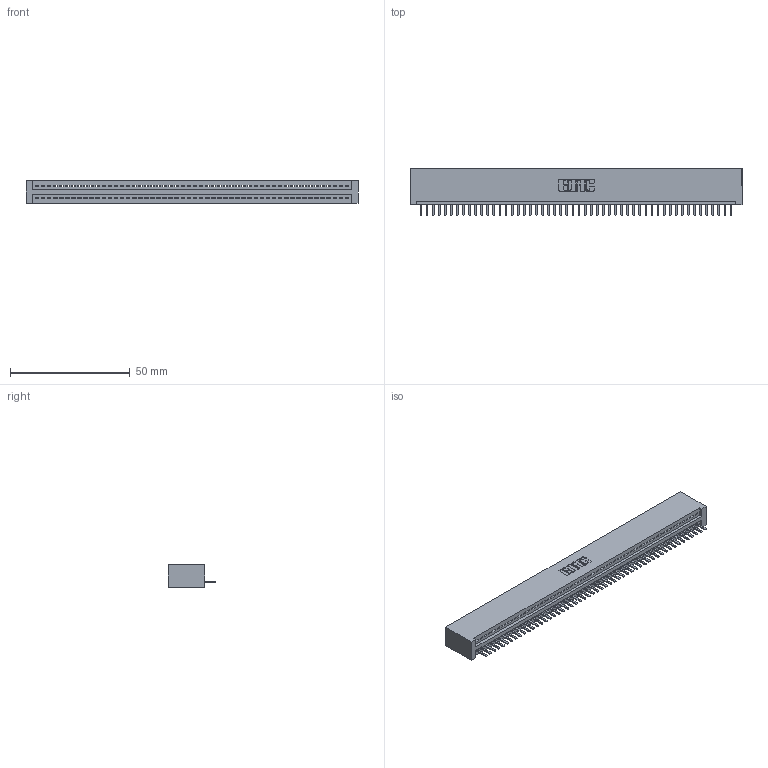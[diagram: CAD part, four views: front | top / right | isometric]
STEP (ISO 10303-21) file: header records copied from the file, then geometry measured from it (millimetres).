
FILE_DESCRIPTION (( 'STEP AP203' ), '1' );
FILE_NAME ('395-052-520-101.STEP', '2019-10-23T11:31:00', ( '' ), ( '' ), 'SwSTEP 2.0', 'SolidWorks 2016', '' );
FILE_SCHEMA (( 'CONFIG_CONTROL_DESIGN' ));
Length unit declared in the file: inch
Products named in the file (3): 345 Part_No Mounting Lugs; 395-052-520-101; 345-292-001_345-293-120
Assembly tree (53 placements, depth 2):
  395-052-520-101
    345 Part_No Mounting Lugs
    345-292-001_345-293-120  x52
Bounding box: 138.68 x 19.68 x 9.4 mm (x, y, z)
Volume: 13689 mm3; surface area: 18028.2 mm2
Topology: 53 solids, 53 shells, 3342 faces, 9885 edges, 6450 vertices
Faces by surface type: plane 2260, cylinder 1082
Entity records: 37627 total; most frequent: CARTESIAN_POINT 6536, ORIENTED_EDGE 6510, DIRECTION 5675, EDGE_CURVE 3255, LINE 2919, VECTOR 2919, VERTEX_POINT 2166, AXIS2_PLACEMENT_3D 1378
